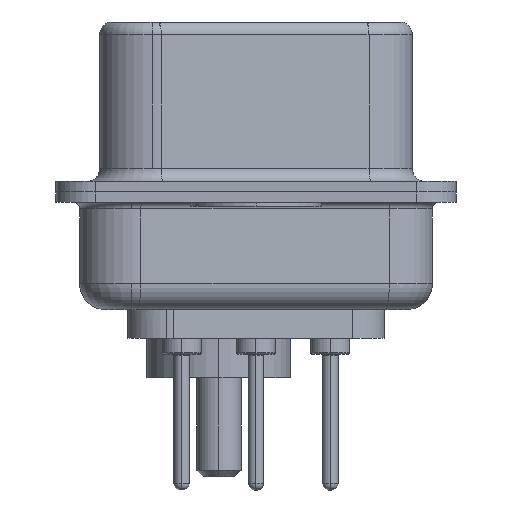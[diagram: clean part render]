
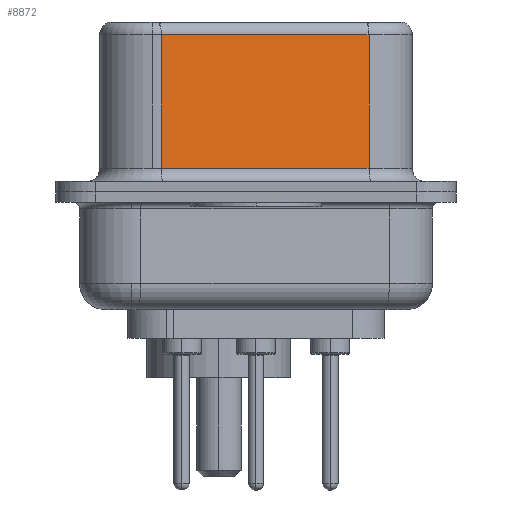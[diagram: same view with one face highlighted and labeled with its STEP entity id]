
A CAD part, left-side view. The second image highlights one B-rep face of the part: STEP entity #8872.
In plain terms, the highlighted planar face has unit normal (-0.985, -0.174, 0).
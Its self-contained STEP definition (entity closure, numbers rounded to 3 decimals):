
#929 = DIRECTION ( 'NONE',  ( -0.174, 0.985, 0. ) ) ;
#1476 = AXIS2_PLACEMENT_3D ( 'NONE', #9376, #13543, #929 ) ;
#2759 = ORIENTED_EDGE ( 'NONE', *, *, #8590, .T. ) ;
#4446 = VECTOR ( 'NONE', #25379, 1000. ) ;
#5225 = PLANE ( 'NONE',  #1476 ) ;
#6173 = VECTOR ( 'NONE', #27062, 1000. ) ;
#6699 = VERTEX_POINT ( 'NONE', #8291 ) ;
#6785 = CARTESIAN_POINT ( 'NONE',  ( 5.132, -4.322, 6.02 ) ) ;
#8291 = CARTESIAN_POINT ( 'NONE',  ( 3.73, 3.628, 6.02 ) ) ;
#8394 = VECTOR ( 'NONE', #11579, 1000. ) ;
#8590 = EDGE_CURVE ( 'NONE', #15683, #6699, #26267, .T. ) ;
#8872 = ADVANCED_FACE ( 'NONE', ( #8992 ), #5225, .F. ) ;
#8892 = EDGE_CURVE ( 'NONE', #15683, #17655, #20150, .T. ) ;
#8992 = FACE_OUTER_BOUND ( 'NONE', #23120, .T. ) ;
#9376 = CARTESIAN_POINT ( 'NONE',  ( 5.132, -4.322, 6.52 ) ) ;
#9454 = CARTESIAN_POINT ( 'NONE',  ( 5.132, -4.322, 6.52 ) ) ;
#9973 = CARTESIAN_POINT ( 'NONE',  ( 5.132, -4.322, 0.9 ) ) ;
#10748 = VECTOR ( 'NONE', #24869, 1000. ) ;
#11120 = EDGE_CURVE ( 'NONE', #26743, #17655, #16324, .T. ) ;
#11579 = DIRECTION ( 'NONE',  ( 0., 0., -1. ) ) ;
#11999 = ORIENTED_EDGE ( 'NONE', *, *, #8892, .F. ) ;
#12157 = CARTESIAN_POINT ( 'NONE',  ( 3.73, 3.628, 6.52 ) ) ;
#12357 = EDGE_CURVE ( 'NONE', #6699, #26743, #22974, .T. ) ;
#13543 = DIRECTION ( 'NONE',  ( 0.985, 0.174, 0. ) ) ;
#15683 = VERTEX_POINT ( 'NONE', #6785 ) ;
#16324 = LINE ( 'NONE', #9973, #10748 ) ;
#17655 = VERTEX_POINT ( 'NONE', #27591 ) ;
#18941 = CARTESIAN_POINT ( 'NONE',  ( 5.132, -4.322, 6.02 ) ) ;
#20150 = LINE ( 'NONE', #9454, #8394 ) ;
#22493 = ORIENTED_EDGE ( 'NONE', *, *, #12357, .T. ) ;
#22974 = LINE ( 'NONE', #12157, #6173 ) ;
#23120 = EDGE_LOOP ( 'NONE', ( #11999, #2759, #22493, #23521 ) ) ;
#23521 = ORIENTED_EDGE ( 'NONE', *, *, #11120, .T. ) ;
#23594 = CARTESIAN_POINT ( 'NONE',  ( 3.73, 3.628, 0.9 ) ) ;
#24869 = DIRECTION ( 'NONE',  ( 0.174, -0.985, 0. ) ) ;
#25379 = DIRECTION ( 'NONE',  ( -0.174, 0.985, 0. ) ) ;
#26267 = LINE ( 'NONE', #18941, #4446 ) ;
#26743 = VERTEX_POINT ( 'NONE', #23594 ) ;
#27062 = DIRECTION ( 'NONE',  ( 0., 0., -1. ) ) ;
#27591 = CARTESIAN_POINT ( 'NONE',  ( 5.132, -4.322, 0.9 ) ) ;
